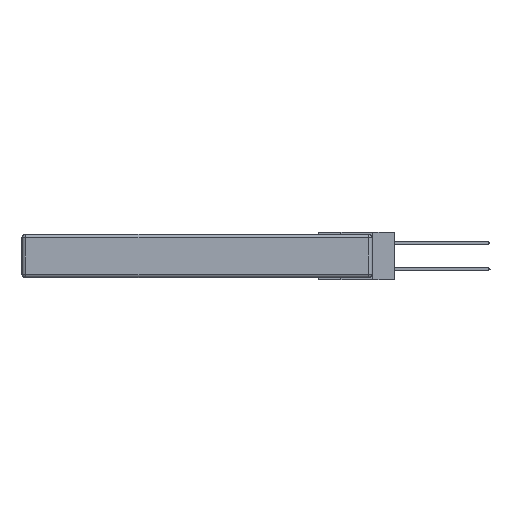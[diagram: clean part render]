
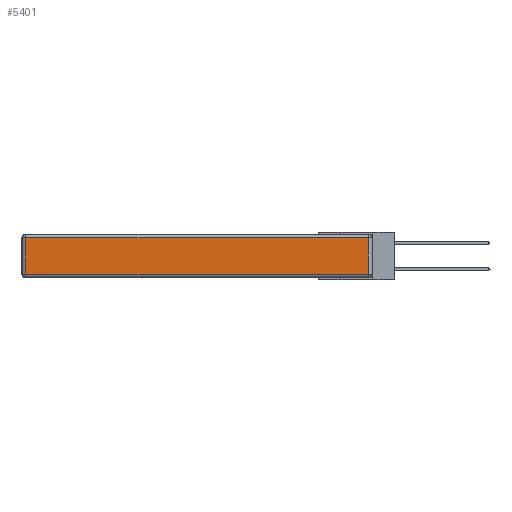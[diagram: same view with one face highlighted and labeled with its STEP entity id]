
A CAD part, left-side view. The second image highlights one B-rep face of the part: STEP entity #5401.
In plain terms, the highlighted planar face has unit normal (-1, 0, 0).
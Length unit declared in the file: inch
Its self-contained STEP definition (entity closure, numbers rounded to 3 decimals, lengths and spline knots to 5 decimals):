
#187 = EDGE_LOOP ( 'NONE', ( #23049, #22069, #9783, #20622 ) ) ;
#239 = DIRECTION ( 'NONE',  ( 0., -1., 0. ) ) ;
#1913 = VECTOR ( 'NONE', #239, 39.37008 ) ;
#2613 = VERTEX_POINT ( 'NONE', #15089 ) ;
#3289 = CARTESIAN_POINT ( 'NONE',  ( 0., 2.72, -0.03 ) ) ;
#3824 = VECTOR ( 'NONE', #6744, 39.37008 ) ;
#3921 = PLANE ( 'NONE',  #4182 ) ;
#4182 = AXIS2_PLACEMENT_3D ( 'NONE', #17038, #5824, #13184 ) ;
#4379 = EDGE_CURVE ( 'NONE', #7671, #2613, #22166, .T. ) ;
#5401 = ADVANCED_FACE ( 'NONE', ( #23839 ), #3921, .T. ) ;
#5449 = CARTESIAN_POINT ( 'NONE',  ( 0., 2.75, -0.03 ) ) ;
#5824 = DIRECTION ( 'NONE',  ( -1., 0., 0. ) ) ;
#5944 = CARTESIAN_POINT ( 'NONE',  ( 0., 2.72, -0.313 ) ) ;
#6744 = DIRECTION ( 'NONE',  ( 0., 0., 1. ) ) ;
#7464 = LINE ( 'NONE', #19367, #18885 ) ;
#7593 = CARTESIAN_POINT ( 'NONE',  ( 0., 0., -0.313 ) ) ;
#7671 = VERTEX_POINT ( 'NONE', #5944 ) ;
#7976 = CARTESIAN_POINT ( 'NONE',  ( 0., 0.03, -0.03 ) ) ;
#9783 = ORIENTED_EDGE ( 'NONE', *, *, #11420, .T. ) ;
#11113 = DIRECTION ( 'NONE',  ( 0., 1., 0. ) ) ;
#11265 = EDGE_CURVE ( 'NONE', #2613, #18313, #15252, .T. ) ;
#11420 = EDGE_CURVE ( 'NONE', #18313, #23121, #16435, .T. ) ;
#12558 = CARTESIAN_POINT ( 'NONE',  ( 0., 0.03, -0.343 ) ) ;
#13184 = DIRECTION ( 'NONE',  ( 0., 0., 1. ) ) ;
#13796 = DIRECTION ( 'NONE',  ( 0., 0., -1. ) ) ;
#15089 = CARTESIAN_POINT ( 'NONE',  ( 0., 0.03, -0.313 ) ) ;
#15228 = VECTOR ( 'NONE', #11113, 39.37008 ) ;
#15252 = LINE ( 'NONE', #12558, #3824 ) ;
#16435 = LINE ( 'NONE', #5449, #15228 ) ;
#17038 = CARTESIAN_POINT ( 'NONE',  ( 0., 0., -0.343 ) ) ;
#17988 = EDGE_CURVE ( 'NONE', #23121, #7671, #7464, .T. ) ;
#18313 = VERTEX_POINT ( 'NONE', #7976 ) ;
#18885 = VECTOR ( 'NONE', #13796, 39.37008 ) ;
#19367 = CARTESIAN_POINT ( 'NONE',  ( 0., 2.72, -0.343 ) ) ;
#20622 = ORIENTED_EDGE ( 'NONE', *, *, #17988, .T. ) ;
#22069 = ORIENTED_EDGE ( 'NONE', *, *, #11265, .T. ) ;
#22166 = LINE ( 'NONE', #7593, #1913 ) ;
#23049 = ORIENTED_EDGE ( 'NONE', *, *, #4379, .T. ) ;
#23121 = VERTEX_POINT ( 'NONE', #3289 ) ;
#23839 = FACE_OUTER_BOUND ( 'NONE', #187, .T. ) ;
